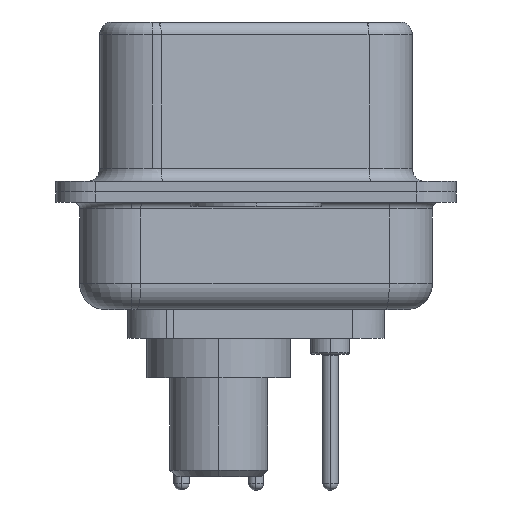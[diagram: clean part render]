
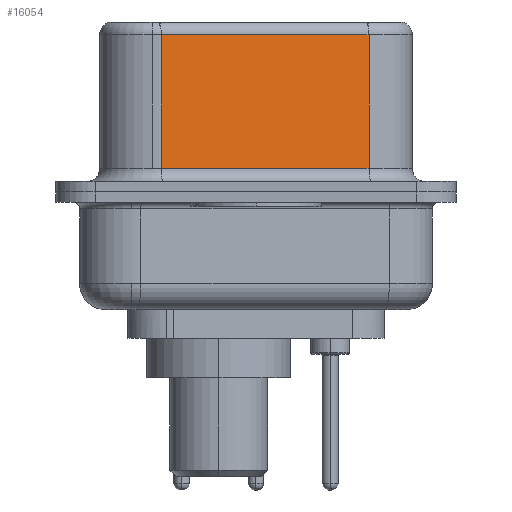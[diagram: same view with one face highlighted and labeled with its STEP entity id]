
A CAD part, left-side view. The second image highlights one B-rep face of the part: STEP entity #16054.
In plain terms, the highlighted planar face has unit normal (-0.985, -0.174, 0).
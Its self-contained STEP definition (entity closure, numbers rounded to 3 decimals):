
#167 = EDGE_CURVE ( 'NONE', #14267, #22927, #7231, .T. ) ;
#196 = ORIENTED_EDGE ( 'NONE', *, *, #13576, .T. ) ;
#638 = CARTESIAN_POINT ( 'NONE',  ( 5.132, -4.322, 0.9 ) ) ;
#1033 = CARTESIAN_POINT ( 'NONE',  ( 5.132, -4.322, 0.9 ) ) ;
#1199 = EDGE_CURVE ( 'NONE', #14267, #3657, #18639, .T. ) ;
#1660 = DIRECTION ( 'NONE',  ( 0., 0., -1. ) ) ;
#1717 = LINE ( 'NONE', #16740, #21212 ) ;
#2094 = VECTOR ( 'NONE', #4855, 1000. ) ;
#2280 = VERTEX_POINT ( 'NONE', #15338 ) ;
#3657 = VERTEX_POINT ( 'NONE', #1033 ) ;
#4061 = DIRECTION ( 'NONE',  ( 0.985, 0.174, 0. ) ) ;
#4413 = CARTESIAN_POINT ( 'NONE',  ( 5.132, -4.322, 6.02 ) ) ;
#4855 = DIRECTION ( 'NONE',  ( 0.174, -0.985, 0. ) ) ;
#6580 = EDGE_CURVE ( 'NONE', #2280, #3657, #7219, .T. ) ;
#6887 = CARTESIAN_POINT ( 'NONE',  ( 3.73, 3.628, 6.02 ) ) ;
#7059 = DIRECTION ( 'NONE',  ( 0., 0., -1. ) ) ;
#7219 = LINE ( 'NONE', #638, #2094 ) ;
#7231 = LINE ( 'NONE', #7657, #21576 ) ;
#7532 = VECTOR ( 'NONE', #7059, 1000. ) ;
#7657 = CARTESIAN_POINT ( 'NONE',  ( 5.132, -4.322, 6.02 ) ) ;
#8013 = DIRECTION ( 'NONE',  ( -0.174, 0.985, 0. ) ) ;
#10717 = CARTESIAN_POINT ( 'NONE',  ( 5.132, -4.322, 6.52 ) ) ;
#11491 = ORIENTED_EDGE ( 'NONE', *, *, #167, .T. ) ;
#13576 = EDGE_CURVE ( 'NONE', #22927, #2280, #1717, .T. ) ;
#14267 = VERTEX_POINT ( 'NONE', #4413 ) ;
#15338 = CARTESIAN_POINT ( 'NONE',  ( 3.73, 3.628, 0.9 ) ) ;
#15359 = PLANE ( 'NONE',  #22537 ) ;
#15626 = ORIENTED_EDGE ( 'NONE', *, *, #6580, .T. ) ;
#15876 = EDGE_LOOP ( 'NONE', ( #16092, #11491, #196, #15626 ) ) ;
#16054 = ADVANCED_FACE ( 'NONE', ( #21688 ), #15359, .F. ) ;
#16092 = ORIENTED_EDGE ( 'NONE', *, *, #1199, .F. ) ;
#16740 = CARTESIAN_POINT ( 'NONE',  ( 3.73, 3.628, 6.52 ) ) ;
#17233 = DIRECTION ( 'NONE',  ( -0.174, 0.985, 0. ) ) ;
#18639 = LINE ( 'NONE', #10717, #7532 ) ;
#20889 = CARTESIAN_POINT ( 'NONE',  ( 5.132, -4.322, 6.52 ) ) ;
#21212 = VECTOR ( 'NONE', #1660, 1000. ) ;
#21576 = VECTOR ( 'NONE', #8013, 1000. ) ;
#21688 = FACE_OUTER_BOUND ( 'NONE', #15876, .T. ) ;
#22537 = AXIS2_PLACEMENT_3D ( 'NONE', #20889, #4061, #17233 ) ;
#22927 = VERTEX_POINT ( 'NONE', #6887 ) ;
